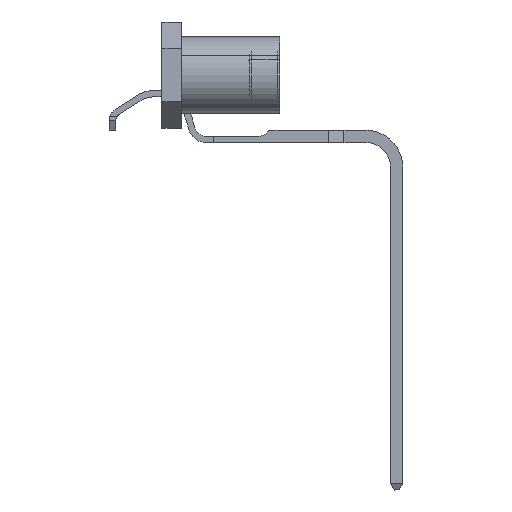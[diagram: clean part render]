
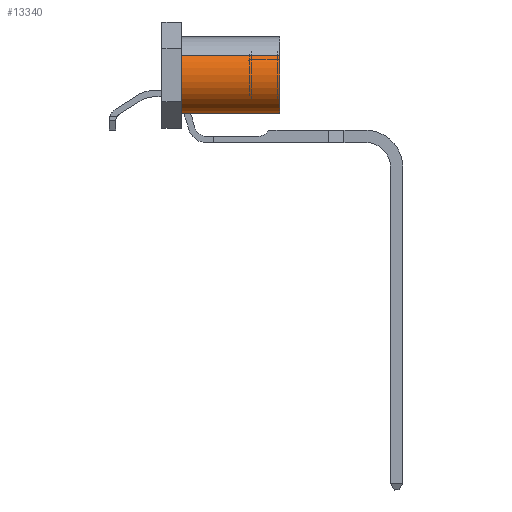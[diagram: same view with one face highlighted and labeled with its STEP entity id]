
A CAD part, left-side view. The second image highlights one B-rep face of the part: STEP entity #13340.
In plain terms, the highlighted cylindrical face has radius 1.968 mm (diameter 3.937 mm), a partial arc.
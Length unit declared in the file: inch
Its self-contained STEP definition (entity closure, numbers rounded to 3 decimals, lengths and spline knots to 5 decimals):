
#433 = DIRECTION ( 'NONE',  ( 0., 0., 1. ) ) ;
#513 = VECTOR ( 'NONE', #3307, 39.37008 ) ;
#557 = EDGE_CURVE ( 'NONE', #11427, #20753, #21020, .T. ) ;
#874 = VERTEX_POINT ( 'NONE', #3466 ) ;
#1074 = CIRCLE ( 'NONE', #20065, 0.0775 ) ;
#1275 = CARTESIAN_POINT ( 'NONE',  ( 0., 0.24, 0. ) ) ;
#1533 = LINE ( 'NONE', #9271, #4992 ) ;
#1656 = DIRECTION ( 'NONE',  ( 0., -1., 0. ) ) ;
#3307 = DIRECTION ( 'NONE',  ( 0., -1., 0. ) ) ;
#3466 = CARTESIAN_POINT ( 'NONE',  ( 0., 0.24, 0.0775 ) ) ;
#3549 = CARTESIAN_POINT ( 'NONE',  ( 0., 0.04, 0. ) ) ;
#3631 = ORIENTED_EDGE ( 'NONE', *, *, #19781, .F. ) ;
#4344 = ORIENTED_EDGE ( 'NONE', *, *, #557, .T. ) ;
#4461 = CARTESIAN_POINT ( 'NONE',  ( 0., 0.24, 0. ) ) ;
#4992 = VECTOR ( 'NONE', #1656, 39.37008 ) ;
#6623 = ORIENTED_EDGE ( 'NONE', *, *, #7936, .F. ) ;
#6994 = AXIS2_PLACEMENT_3D ( 'NONE', #1275, #13519, #24925 ) ;
#7517 = CARTESIAN_POINT ( 'NONE',  ( 0., 0.04, 0.0775 ) ) ;
#7767 = CIRCLE ( 'NONE', #23063, 0.0775 ) ;
#7936 = EDGE_CURVE ( 'NONE', #11427, #874, #7767, .T. ) ;
#9271 = CARTESIAN_POINT ( 'NONE',  ( 0., 0.24, 0.0775 ) ) ;
#9579 = DIRECTION ( 'NONE',  ( 0., 1., 0. ) ) ;
#11044 = FACE_OUTER_BOUND ( 'NONE', #18183, .T. ) ;
#11427 = VERTEX_POINT ( 'NONE', #14334 ) ;
#13340 = ADVANCED_FACE ( 'NONE', ( #11044 ), #18979, .T. ) ;
#13519 = DIRECTION ( 'NONE',  ( 0., -1., 0. ) ) ;
#14108 = VERTEX_POINT ( 'NONE', #7517 ) ;
#14334 = CARTESIAN_POINT ( 'NONE',  ( 0., 0.24, -0.0775 ) ) ;
#15104 = ORIENTED_EDGE ( 'NONE', *, *, #15557, .T. ) ;
#15262 = CARTESIAN_POINT ( 'NONE',  ( 0., 0.04, -0.0775 ) ) ;
#15557 = EDGE_CURVE ( 'NONE', #20753, #14108, #1074, .T. ) ;
#15889 = DIRECTION ( 'NONE',  ( 0., 0., 1. ) ) ;
#16449 = CARTESIAN_POINT ( 'NONE',  ( 0., 0.24, -0.0775 ) ) ;
#18183 = EDGE_LOOP ( 'NONE', ( #3631, #6623, #4344, #15104 ) ) ;
#18979 = CYLINDRICAL_SURFACE ( 'NONE', #6994, 0.0775 ) ;
#19781 = EDGE_CURVE ( 'NONE', #874, #14108, #1533, .T. ) ;
#19828 = DIRECTION ( 'NONE',  ( 0., 1., 0. ) ) ;
#20065 = AXIS2_PLACEMENT_3D ( 'NONE', #3549, #9579, #15889 ) ;
#20753 = VERTEX_POINT ( 'NONE', #15262 ) ;
#21020 = LINE ( 'NONE', #16449, #513 ) ;
#23063 = AXIS2_PLACEMENT_3D ( 'NONE', #4461, #19828, #433 ) ;
#24925 = DIRECTION ( 'NONE',  ( 0., 0., -1. ) ) ;
